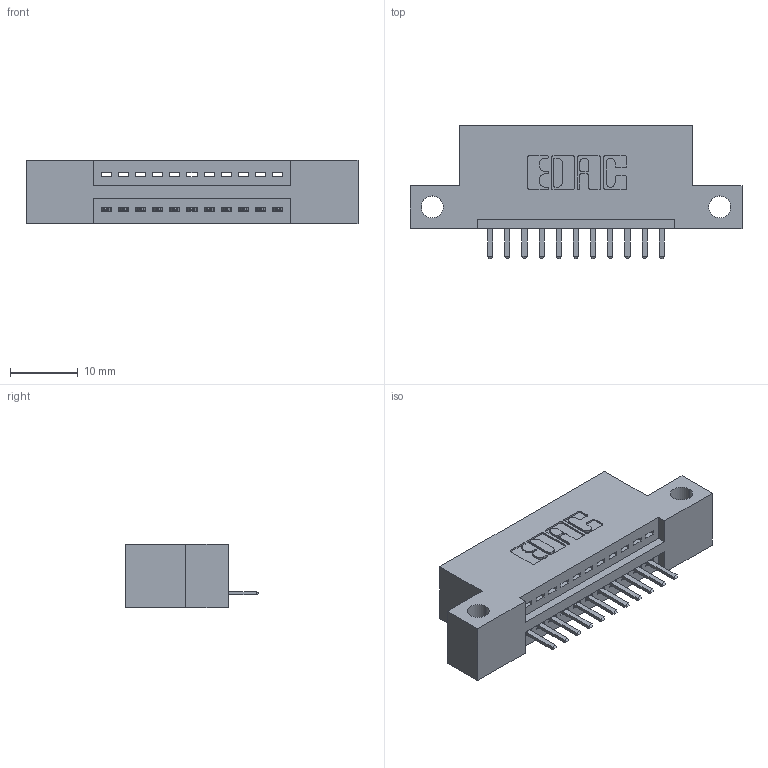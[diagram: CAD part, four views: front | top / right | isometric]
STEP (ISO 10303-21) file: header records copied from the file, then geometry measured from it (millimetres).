
FILE_DESCRIPTION (( 'STEP AP203' ), '1' );
FILE_NAME ('345-011-520-112.STEP', '2018-08-17T22:45:48', ( '' ), ( '' ), 'SwSTEP 2.0', 'SolidWorks 2016', '' );
FILE_SCHEMA (( 'CONFIG_CONTROL_DESIGN' ));
Length unit declared in the file: inch
Products named in the file (3): 345-292-001_345-293-120; 345-011-520-112; 345 Part_Flush Mounting Lugs - Side Mount
Assembly tree (12 placements, depth 2):
  345-011-520-112
    345 Part_Flush Mounting Lugs - Side Mount
    345-292-001_345-293-120  x11
Bounding box: 49.15 x 19.68 x 9.4 mm (x, y, z)
Volume: 4295.3 mm3; surface area: 5041.3 mm2
Topology: 12 solids, 12 shells, 808 faces, 2365 edges, 1546 vertices
Faces by surface type: plane 542, cylinder 266
Entity records: 12569 total; most frequent: CARTESIAN_POINT 2197, ORIENTED_EDGE 2130, DIRECTION 1951, EDGE_CURVE 1065, LINE 885, VECTOR 885, VERTEX_POINT 706, AXIS2_PLACEMENT_3D 533
